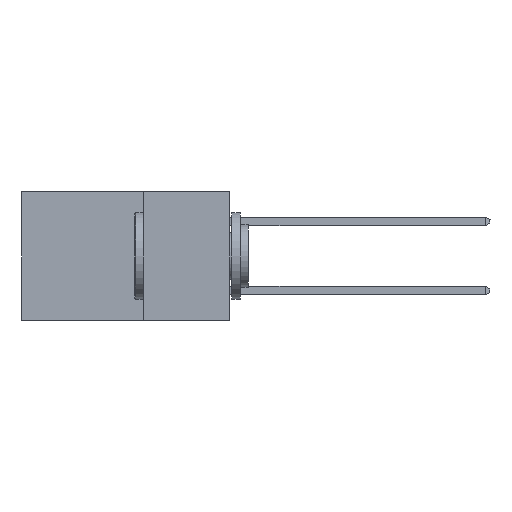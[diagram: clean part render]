
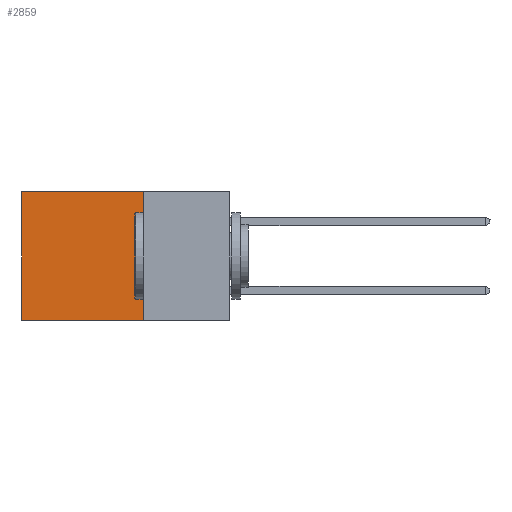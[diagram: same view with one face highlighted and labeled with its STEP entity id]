
A CAD part, left-side view. The second image highlights one B-rep face of the part: STEP entity #2859.
In plain terms, the highlighted planar face has unit normal (-1, 0, 0).
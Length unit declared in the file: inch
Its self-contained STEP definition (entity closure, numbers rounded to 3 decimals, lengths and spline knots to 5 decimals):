
#299 = DIRECTION ( 'NONE',  ( 0., 0., -1. ) ) ;
#370 = PLANE ( 'NONE',  #23727 ) ;
#924 = VECTOR ( 'NONE', #8529, 39.37008 ) ;
#2428 = DIRECTION ( 'NONE',  ( 1., 0., 0. ) ) ;
#2859 = ADVANCED_FACE ( 'NONE', ( #17286 ), #370, .F. ) ;
#2963 = VECTOR ( 'NONE', #299, 39.37008 ) ;
#3256 = VERTEX_POINT ( 'NONE', #17763 ) ;
#4698 = ORIENTED_EDGE ( 'NONE', *, *, #25411, .F. ) ;
#5552 = CARTESIAN_POINT ( 'NONE',  ( 0.2615, 0.25, -0.37 ) ) ;
#6130 = EDGE_LOOP ( 'NONE', ( #16133, #17158, #4698, #22303 ) ) ;
#7462 = CARTESIAN_POINT ( 'NONE',  ( 0.2615, 0.25, -0.37 ) ) ;
#7944 = CARTESIAN_POINT ( 'NONE',  ( 0.2615, 0.25, 0. ) ) ;
#8212 = DIRECTION ( 'NONE',  ( 0., 0., -1. ) ) ;
#8529 = DIRECTION ( 'NONE',  ( 0., 0., -1. ) ) ;
#8613 = DIRECTION ( 'NONE',  ( 0., 1., 0. ) ) ;
#8831 = EDGE_CURVE ( 'NONE', #14534, #23183, #9738, .T. ) ;
#9738 = LINE ( 'NONE', #7944, #11343 ) ;
#11010 = VECTOR ( 'NONE', #8613, 39.37008 ) ;
#11343 = VECTOR ( 'NONE', #13877, 39.37008 ) ;
#12021 = LINE ( 'NONE', #19887, #2963 ) ;
#12400 = CARTESIAN_POINT ( 'NONE',  ( 0.2615, 0.25, -0.37 ) ) ;
#13144 = EDGE_CURVE ( 'NONE', #18436, #3256, #20474, .T. ) ;
#13235 = CARTESIAN_POINT ( 'NONE',  ( 0.2615, 0.6, 0. ) ) ;
#13877 = DIRECTION ( 'NONE',  ( 0., 1., 0. ) ) ;
#14534 = VERTEX_POINT ( 'NONE', #20284 ) ;
#16133 = ORIENTED_EDGE ( 'NONE', *, *, #25236, .T. ) ;
#17158 = ORIENTED_EDGE ( 'NONE', *, *, #13144, .F. ) ;
#17286 = FACE_OUTER_BOUND ( 'NONE', #6130, .T. ) ;
#17763 = CARTESIAN_POINT ( 'NONE',  ( 0.2615, 0.6, -0.37 ) ) ;
#18436 = VERTEX_POINT ( 'NONE', #7462 ) ;
#19887 = CARTESIAN_POINT ( 'NONE',  ( 0.2615, 0.6, -0.37 ) ) ;
#20284 = CARTESIAN_POINT ( 'NONE',  ( 0.2615, 0.25, 0. ) ) ;
#20474 = LINE ( 'NONE', #22411, #11010 ) ;
#22221 = LINE ( 'NONE', #12400, #924 ) ;
#22303 = ORIENTED_EDGE ( 'NONE', *, *, #8831, .T. ) ;
#22411 = CARTESIAN_POINT ( 'NONE',  ( 0.2615, 0.25, -0.37 ) ) ;
#23183 = VERTEX_POINT ( 'NONE', #13235 ) ;
#23727 = AXIS2_PLACEMENT_3D ( 'NONE', #5552, #2428, #8212 ) ;
#25236 = EDGE_CURVE ( 'NONE', #23183, #3256, #12021, .T. ) ;
#25411 = EDGE_CURVE ( 'NONE', #14534, #18436, #22221, .T. ) ;
